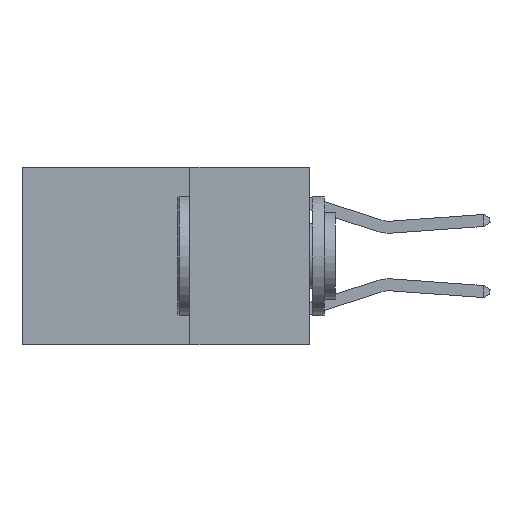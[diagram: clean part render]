
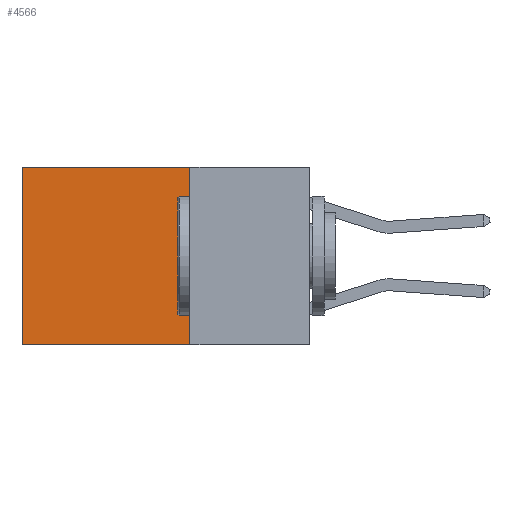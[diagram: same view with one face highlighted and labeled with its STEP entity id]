
A CAD part, left-side view. The second image highlights one B-rep face of the part: STEP entity #4566.
In plain terms, the highlighted planar face has unit normal (-1, 0, 0).
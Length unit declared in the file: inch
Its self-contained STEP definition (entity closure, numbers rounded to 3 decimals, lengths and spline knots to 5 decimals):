
#36 = AXIS2_PLACEMENT_3D ( 'NONE', #16477, #6181, #2042 ) ;
#675 = CARTESIAN_POINT ( 'NONE',  ( 0.2625, 0.25, 0. ) ) ;
#1645 = EDGE_CURVE ( 'NONE', #5306, #10792, #9851, .T. ) ;
#2042 = DIRECTION ( 'NONE',  ( 0., 0., -1. ) ) ;
#2127 = FACE_OUTER_BOUND ( 'NONE', #12892, .T. ) ;
#2443 = LINE ( 'NONE', #10405, #15477 ) ;
#3267 = LINE ( 'NONE', #5895, #10763 ) ;
#3420 = CARTESIAN_POINT ( 'NONE',  ( 0.2625, 0.25, 0. ) ) ;
#3518 = ORIENTED_EDGE ( 'NONE', *, *, #1645, .F. ) ;
#4381 = CARTESIAN_POINT ( 'NONE',  ( 0.2625, 0.6, -0.37 ) ) ;
#4411 = LINE ( 'NONE', #675, #13632 ) ;
#4566 = ADVANCED_FACE ( 'NONE', ( #2127 ), #7534, .F. ) ;
#5306 = VERTEX_POINT ( 'NONE', #3420 ) ;
#5584 = CARTESIAN_POINT ( 'NONE',  ( 0.2625, 0.25, -0.37 ) ) ;
#5693 = DIRECTION ( 'NONE',  ( 0., 1., 0. ) ) ;
#5895 = CARTESIAN_POINT ( 'NONE',  ( 0.2625, 0.25, -0.37 ) ) ;
#6181 = DIRECTION ( 'NONE',  ( 1., 0., 0. ) ) ;
#6475 = CARTESIAN_POINT ( 'NONE',  ( 0.2625, 0.6, 0. ) ) ;
#6697 = VERTEX_POINT ( 'NONE', #6475 ) ;
#6993 = ORIENTED_EDGE ( 'NONE', *, *, #9022, .T. ) ;
#7534 = PLANE ( 'NONE',  #36 ) ;
#8153 = ORIENTED_EDGE ( 'NONE', *, *, #13767, .F. ) ;
#9022 = EDGE_CURVE ( 'NONE', #5306, #6697, #4411, .T. ) ;
#9607 = CARTESIAN_POINT ( 'NONE',  ( 0.2625, 0.25, 0. ) ) ;
#9851 = LINE ( 'NONE', #9607, #14459 ) ;
#10405 = CARTESIAN_POINT ( 'NONE',  ( 0.2625, 0.6, 0. ) ) ;
#10763 = VECTOR ( 'NONE', #12388, 39.37008 ) ;
#10792 = VERTEX_POINT ( 'NONE', #5584 ) ;
#11055 = EDGE_CURVE ( 'NONE', #6697, #11855, #2443, .T. ) ;
#11855 = VERTEX_POINT ( 'NONE', #4381 ) ;
#12369 = DIRECTION ( 'NONE',  ( 0., 0., -1. ) ) ;
#12388 = DIRECTION ( 'NONE',  ( 0., 1., 0. ) ) ;
#12892 = EDGE_LOOP ( 'NONE', ( #15650, #8153, #3518, #6993 ) ) ;
#13632 = VECTOR ( 'NONE', #5693, 39.37008 ) ;
#13767 = EDGE_CURVE ( 'NONE', #10792, #11855, #3267, .T. ) ;
#14459 = VECTOR ( 'NONE', #12369, 39.37008 ) ;
#15477 = VECTOR ( 'NONE', #15527, 39.37008 ) ;
#15527 = DIRECTION ( 'NONE',  ( 0., 0., -1. ) ) ;
#15650 = ORIENTED_EDGE ( 'NONE', *, *, #11055, .T. ) ;
#16477 = CARTESIAN_POINT ( 'NONE',  ( 0.2625, 0.25, 0. ) ) ;
